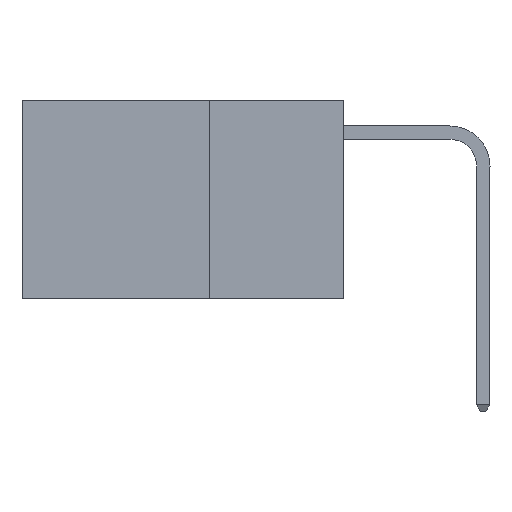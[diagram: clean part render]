
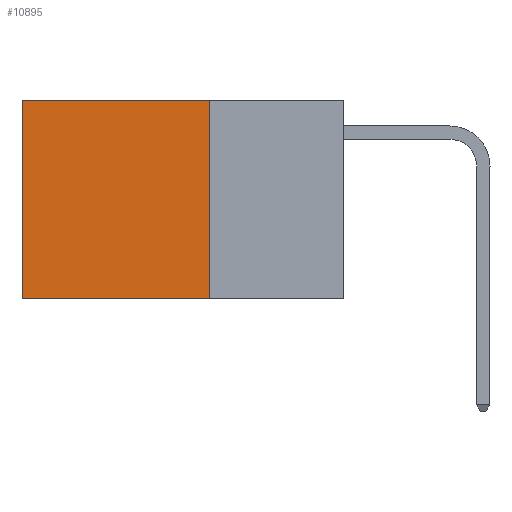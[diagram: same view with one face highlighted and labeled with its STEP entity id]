
A CAD part, left-side view. The second image highlights one B-rep face of the part: STEP entity #10895.
In plain terms, the highlighted planar face has unit normal (-1, 0, 0).
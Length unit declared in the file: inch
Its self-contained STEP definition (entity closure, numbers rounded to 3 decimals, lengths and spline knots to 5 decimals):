
#896 = VECTOR ( 'NONE', #3786, 39.37008 ) ;
#1052 = VECTOR ( 'NONE', #2951, 39.37008 ) ;
#1296 = DIRECTION ( 'NONE',  ( 0., 0., -1. ) ) ;
#1508 = CARTESIAN_POINT ( 'NONE',  ( 0.2625, 0.6, 0. ) ) ;
#1986 = EDGE_LOOP ( 'NONE', ( #8072, #8085, #8215, #8345 ) ) ;
#2482 = CARTESIAN_POINT ( 'NONE',  ( 0.2625, 0.6, -0.37 ) ) ;
#2951 = DIRECTION ( 'NONE',  ( 0., 1., 0. ) ) ;
#3611 = EDGE_CURVE ( 'NONE', #12358, #5078, #6333, .T. ) ;
#3786 = DIRECTION ( 'NONE',  ( 0., 0., -1. ) ) ;
#3858 = EDGE_CURVE ( 'NONE', #10435, #5078, #12520, .T. ) ;
#4145 = DIRECTION ( 'NONE',  ( 0., 0., -1. ) ) ;
#4504 = CARTESIAN_POINT ( 'NONE',  ( 0.2625, 0.25, -0.37 ) ) ;
#4779 = CARTESIAN_POINT ( 'NONE',  ( 0.2625, 0.25, 0. ) ) ;
#5078 = VERTEX_POINT ( 'NONE', #2482 ) ;
#6054 = VERTEX_POINT ( 'NONE', #6117 ) ;
#6117 = CARTESIAN_POINT ( 'NONE',  ( 0.2625, 0.25, 0. ) ) ;
#6154 = LINE ( 'NONE', #4779, #896 ) ;
#6169 = FACE_OUTER_BOUND ( 'NONE', #1986, .T. ) ;
#6304 = LINE ( 'NONE', #11558, #1052 ) ;
#6333 = LINE ( 'NONE', #1508, #11109 ) ;
#7009 = PLANE ( 'NONE',  #7041 ) ;
#7041 = AXIS2_PLACEMENT_3D ( 'NONE', #8939, #9892, #4145 ) ;
#7571 = VECTOR ( 'NONE', #10839, 39.37008 ) ;
#8072 = ORIENTED_EDGE ( 'NONE', *, *, #3611, .T. ) ;
#8085 = ORIENTED_EDGE ( 'NONE', *, *, #3858, .F. ) ;
#8215 = ORIENTED_EDGE ( 'NONE', *, *, #11351, .F. ) ;
#8345 = ORIENTED_EDGE ( 'NONE', *, *, #12329, .T. ) ;
#8939 = CARTESIAN_POINT ( 'NONE',  ( 0.2625, 0.25, 0. ) ) ;
#9892 = DIRECTION ( 'NONE',  ( 1., 0., 0. ) ) ;
#10435 = VERTEX_POINT ( 'NONE', #4504 ) ;
#10839 = DIRECTION ( 'NONE',  ( 0., 1., 0. ) ) ;
#10865 = CARTESIAN_POINT ( 'NONE',  ( 0.2625, 0.25, -0.37 ) ) ;
#10895 = ADVANCED_FACE ( 'NONE', ( #6169 ), #7009, .F. ) ;
#11109 = VECTOR ( 'NONE', #1296, 39.37008 ) ;
#11351 = EDGE_CURVE ( 'NONE', #6054, #10435, #6154, .T. ) ;
#11558 = CARTESIAN_POINT ( 'NONE',  ( 0.2625, 0.25, 0. ) ) ;
#11597 = CARTESIAN_POINT ( 'NONE',  ( 0.2625, 0.6, 0. ) ) ;
#12329 = EDGE_CURVE ( 'NONE', #6054, #12358, #6304, .T. ) ;
#12358 = VERTEX_POINT ( 'NONE', #11597 ) ;
#12520 = LINE ( 'NONE', #10865, #7571 ) ;
